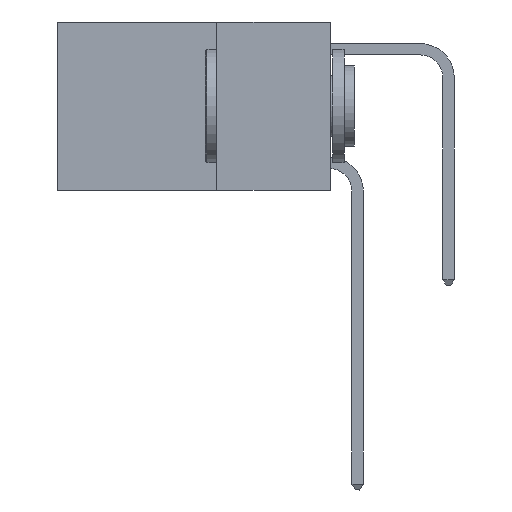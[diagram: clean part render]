
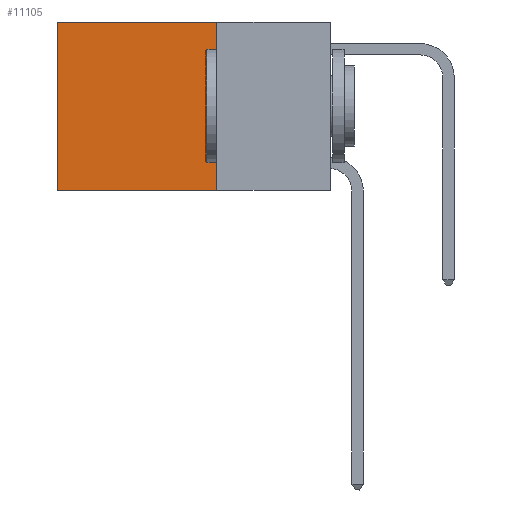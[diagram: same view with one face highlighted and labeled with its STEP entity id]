
A CAD part, left-side view. The second image highlights one B-rep face of the part: STEP entity #11105.
In plain terms, the highlighted planar face has unit normal (-1, 0, 0).
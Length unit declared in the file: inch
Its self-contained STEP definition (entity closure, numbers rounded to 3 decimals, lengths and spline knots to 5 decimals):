
#639 = VECTOR ( 'NONE', #11213, 39.37008 ) ;
#1781 = VERTEX_POINT ( 'NONE', #19438 ) ;
#2549 = EDGE_CURVE ( 'NONE', #13320, #1781, #19354, .T. ) ;
#3008 = ORIENTED_EDGE ( 'NONE', *, *, #4147, .T. ) ;
#3191 = PLANE ( 'NONE',  #4285 ) ;
#3635 = LINE ( 'NONE', #5090, #22618 ) ;
#4063 = DIRECTION ( 'NONE',  ( 0., 0., -1. ) ) ;
#4147 = EDGE_CURVE ( 'NONE', #1781, #22068, #16742, .T. ) ;
#4154 = CARTESIAN_POINT ( 'NONE',  ( 0.2625, 0.25, 0. ) ) ;
#4285 = AXIS2_PLACEMENT_3D ( 'NONE', #21089, #10342, #22858 ) ;
#5090 = CARTESIAN_POINT ( 'NONE',  ( 0.2625, 0.25, -0.37 ) ) ;
#5093 = VECTOR ( 'NONE', #21401, 39.37008 ) ;
#5190 = CARTESIAN_POINT ( 'NONE',  ( 0.2625, 0.25, -0.37 ) ) ;
#7117 = CARTESIAN_POINT ( 'NONE',  ( 0.2625, 0.25, 0. ) ) ;
#7251 = VECTOR ( 'NONE', #4063, 39.37008 ) ;
#7779 = ORIENTED_EDGE ( 'NONE', *, *, #16451, .F. ) ;
#8067 = EDGE_CURVE ( 'NONE', #13320, #17887, #14924, .T. ) ;
#8325 = ORIENTED_EDGE ( 'NONE', *, *, #8067, .F. ) ;
#10342 = DIRECTION ( 'NONE',  ( 1., 0., 0. ) ) ;
#11105 = ADVANCED_FACE ( 'NONE', ( #11972 ), #3191, .F. ) ;
#11213 = DIRECTION ( 'NONE',  ( 0., 0., -1. ) ) ;
#11443 = CARTESIAN_POINT ( 'NONE',  ( 0.2625, 0.25, 0. ) ) ;
#11972 = FACE_OUTER_BOUND ( 'NONE', #21837, .T. ) ;
#12153 = DIRECTION ( 'NONE',  ( 0., 1., 0. ) ) ;
#13320 = VERTEX_POINT ( 'NONE', #11443 ) ;
#14924 = LINE ( 'NONE', #4154, #639 ) ;
#16451 = EDGE_CURVE ( 'NONE', #17887, #22068, #3635, .T. ) ;
#16742 = LINE ( 'NONE', #18363, #7251 ) ;
#17849 = ORIENTED_EDGE ( 'NONE', *, *, #2549, .T. ) ;
#17887 = VERTEX_POINT ( 'NONE', #5190 ) ;
#18363 = CARTESIAN_POINT ( 'NONE',  ( 0.2625, 0.6, 0. ) ) ;
#19354 = LINE ( 'NONE', #7117, #5093 ) ;
#19438 = CARTESIAN_POINT ( 'NONE',  ( 0.2625, 0.6, 0. ) ) ;
#20607 = CARTESIAN_POINT ( 'NONE',  ( 0.2625, 0.6, -0.37 ) ) ;
#21089 = CARTESIAN_POINT ( 'NONE',  ( 0.2625, 0.25, 0. ) ) ;
#21401 = DIRECTION ( 'NONE',  ( 0., 1., 0. ) ) ;
#21837 = EDGE_LOOP ( 'NONE', ( #3008, #7779, #8325, #17849 ) ) ;
#22068 = VERTEX_POINT ( 'NONE', #20607 ) ;
#22618 = VECTOR ( 'NONE', #12153, 39.37008 ) ;
#22858 = DIRECTION ( 'NONE',  ( 0., 0., -1. ) ) ;
